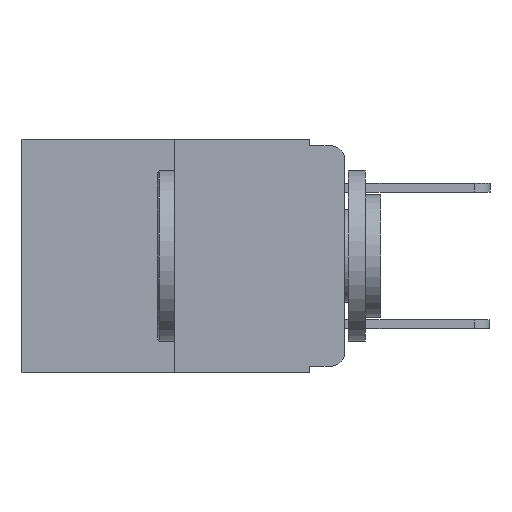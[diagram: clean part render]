
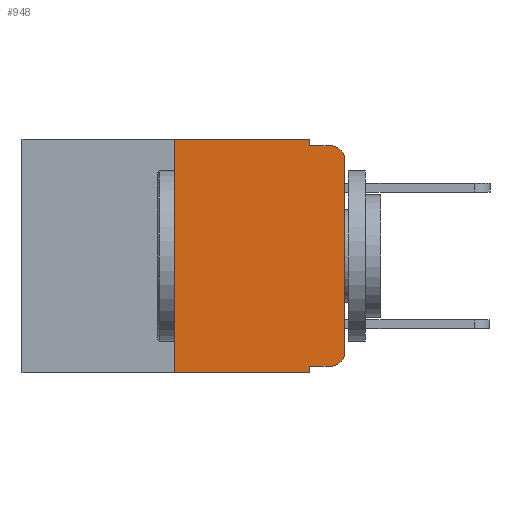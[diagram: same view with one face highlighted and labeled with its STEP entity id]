
A CAD part, left-side view. The second image highlights one B-rep face of the part: STEP entity #948.
In plain terms, the highlighted planar face has unit normal (-1, 0, 0).
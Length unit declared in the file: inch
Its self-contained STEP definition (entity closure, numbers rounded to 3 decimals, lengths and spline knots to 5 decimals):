
#57 = CIRCLE ( 'NONE', #8454, 0.02 ) ;
#77 = PLANE ( 'NONE',  #911 ) ;
#212 = CARTESIAN_POINT ( 'NONE',  ( 0., 0.051, -0.333 ) ) ;
#233 = EDGE_LOOP ( 'NONE', ( #4092, #9973, #11963, #1810, #4814, #7683, #2192, #12409, #2564, #5504 ) ) ;
#443 = CARTESIAN_POINT ( 'NONE',  ( 0., 0.051, -0.01 ) ) ;
#911 = AXIS2_PLACEMENT_3D ( 'NONE', #11942, #3905, #11598 ) ;
#948 = ADVANCED_FACE ( 'NONE', ( #7847 ), #77, .F. ) ;
#1107 = CARTESIAN_POINT ( 'NONE',  ( 0., 0.25, 0. ) ) ;
#1314 = VERTEX_POINT ( 'NONE', #2689 ) ;
#1489 = VERTEX_POINT ( 'NONE', #212 ) ;
#1530 = VERTEX_POINT ( 'NONE', #5446 ) ;
#1761 = EDGE_CURVE ( 'NONE', #1314, #10111, #6148, .T. ) ;
#1810 = ORIENTED_EDGE ( 'NONE', *, *, #1761, .F. ) ;
#1948 = EDGE_CURVE ( 'NONE', #10111, #2426, #10567, .T. ) ;
#2192 = ORIENTED_EDGE ( 'NONE', *, *, #2713, .T. ) ;
#2426 = VERTEX_POINT ( 'NONE', #12488 ) ;
#2473 = VERTEX_POINT ( 'NONE', #3616 ) ;
#2532 = EDGE_CURVE ( 'NONE', #8817, #5841, #10547, .T. ) ;
#2564 = ORIENTED_EDGE ( 'NONE', *, *, #2692, .T. ) ;
#2689 = CARTESIAN_POINT ( 'NONE',  ( 0., 0.051, 0. ) ) ;
#2692 = EDGE_CURVE ( 'NONE', #1489, #8817, #3216, .T. ) ;
#2713 = EDGE_CURVE ( 'NONE', #5913, #2473, #12587, .T. ) ;
#2768 = EDGE_CURVE ( 'NONE', #1489, #2473, #10430, .T. ) ;
#2860 = DIRECTION ( 'NONE',  ( -1., 0., 0. ) ) ;
#3216 = LINE ( 'NONE', #8367, #10896 ) ;
#3405 = CARTESIAN_POINT ( 'NONE',  ( 0., 0.25, -0.343 ) ) ;
#3616 = CARTESIAN_POINT ( 'NONE',  ( 0., 0.051, -0.343 ) ) ;
#3638 = DIRECTION ( 'NONE',  ( 0., -1., 0. ) ) ;
#3905 = DIRECTION ( 'NONE',  ( 1., 0., 0. ) ) ;
#4092 = ORIENTED_EDGE ( 'NONE', *, *, #4455, .T. ) ;
#4405 = CARTESIAN_POINT ( 'NONE',  ( 0., 0., -0.313 ) ) ;
#4455 = EDGE_CURVE ( 'NONE', #5841, #9994, #10268, .T. ) ;
#4814 = ORIENTED_EDGE ( 'NONE', *, *, #5514, .F. ) ;
#5126 = DIRECTION ( 'NONE',  ( 0., 0., -1. ) ) ;
#5209 = EDGE_CURVE ( 'NONE', #9994, #2426, #57, .T. ) ;
#5274 = CARTESIAN_POINT ( 'NONE',  ( 0., 0.051, -0.01 ) ) ;
#5300 = CARTESIAN_POINT ( 'NONE',  ( 0., 0.473, -0.343 ) ) ;
#5446 = CARTESIAN_POINT ( 'NONE',  ( 0., 0.25, 0. ) ) ;
#5447 = VECTOR ( 'NONE', #6415, 39.37008 ) ;
#5504 = ORIENTED_EDGE ( 'NONE', *, *, #2532, .T. ) ;
#5514 = EDGE_CURVE ( 'NONE', #1530, #1314, #9265, .T. ) ;
#5841 = VERTEX_POINT ( 'NONE', #4405 ) ;
#5913 = VERTEX_POINT ( 'NONE', #3405 ) ;
#6148 = LINE ( 'NONE', #10329, #8301 ) ;
#6205 = DIRECTION ( 'NONE',  ( 0., -1., 0. ) ) ;
#6295 = CARTESIAN_POINT ( 'NONE',  ( 0., 0., -0.03 ) ) ;
#6415 = DIRECTION ( 'NONE',  ( 0., -1., 0. ) ) ;
#6464 = AXIS2_PLACEMENT_3D ( 'NONE', #12508, #8867, #8843 ) ;
#6493 = VECTOR ( 'NONE', #3638, 39.37008 ) ;
#6863 = CARTESIAN_POINT ( 'NONE',  ( 0., 0.02, -0.333 ) ) ;
#6874 = CARTESIAN_POINT ( 'NONE',  ( 0., 0.473, 0. ) ) ;
#7626 = VECTOR ( 'NONE', #5126, 39.37008 ) ;
#7683 = ORIENTED_EDGE ( 'NONE', *, *, #8725, .F. ) ;
#7847 = FACE_OUTER_BOUND ( 'NONE', #233, .T. ) ;
#8034 = DIRECTION ( 'NONE',  ( 0., -1., 0. ) ) ;
#8301 = VECTOR ( 'NONE', #8575, 39.37008 ) ;
#8367 = CARTESIAN_POINT ( 'NONE',  ( 0., 0.051, -0.333 ) ) ;
#8454 = AXIS2_PLACEMENT_3D ( 'NONE', #9229, #2860, #10141 ) ;
#8575 = DIRECTION ( 'NONE',  ( 0., 0., -1. ) ) ;
#8725 = EDGE_CURVE ( 'NONE', #5913, #1530, #8740, .T. ) ;
#8740 = LINE ( 'NONE', #1107, #10790 ) ;
#8817 = VERTEX_POINT ( 'NONE', #6863 ) ;
#8843 = DIRECTION ( 'NONE',  ( 0., 0., -1. ) ) ;
#8867 = DIRECTION ( 'NONE',  ( -1., 0., 0. ) ) ;
#9229 = CARTESIAN_POINT ( 'NONE',  ( 0., 0.02, -0.03 ) ) ;
#9265 = LINE ( 'NONE', #6874, #6493 ) ;
#9735 = DIRECTION ( 'NONE',  ( 0., 0., 1. ) ) ;
#9973 = ORIENTED_EDGE ( 'NONE', *, *, #5209, .T. ) ;
#9994 = VERTEX_POINT ( 'NONE', #6295 ) ;
#10022 = VECTOR ( 'NONE', #10271, 39.37008 ) ;
#10111 = VERTEX_POINT ( 'NONE', #5274 ) ;
#10141 = DIRECTION ( 'NONE',  ( 0., 0., -1. ) ) ;
#10268 = LINE ( 'NONE', #10485, #10022 ) ;
#10271 = DIRECTION ( 'NONE',  ( 0., 0., 1. ) ) ;
#10329 = CARTESIAN_POINT ( 'NONE',  ( 0., 0.051, 0. ) ) ;
#10331 = VECTOR ( 'NONE', #8034, 39.37008 ) ;
#10430 = LINE ( 'NONE', #11510, #7626 ) ;
#10485 = CARTESIAN_POINT ( 'NONE',  ( 0., 0., 0. ) ) ;
#10547 = CIRCLE ( 'NONE', #6464, 0.02 ) ;
#10567 = LINE ( 'NONE', #443, #10331 ) ;
#10790 = VECTOR ( 'NONE', #9735, 39.37008 ) ;
#10896 = VECTOR ( 'NONE', #6205, 39.37008 ) ;
#11510 = CARTESIAN_POINT ( 'NONE',  ( 0., 0.051, 0. ) ) ;
#11598 = DIRECTION ( 'NONE',  ( 0., 0., -1. ) ) ;
#11942 = CARTESIAN_POINT ( 'NONE',  ( 0., 0.473, 0. ) ) ;
#11963 = ORIENTED_EDGE ( 'NONE', *, *, #1948, .F. ) ;
#12409 = ORIENTED_EDGE ( 'NONE', *, *, #2768, .F. ) ;
#12488 = CARTESIAN_POINT ( 'NONE',  ( 0., 0.02, -0.01 ) ) ;
#12508 = CARTESIAN_POINT ( 'NONE',  ( 0., 0.02, -0.313 ) ) ;
#12587 = LINE ( 'NONE', #5300, #5447 ) ;
